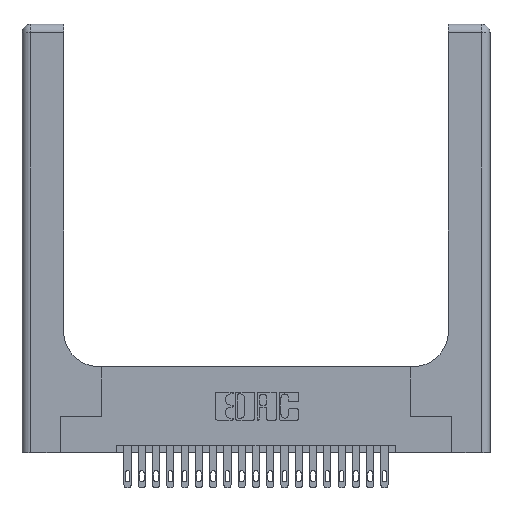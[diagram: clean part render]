
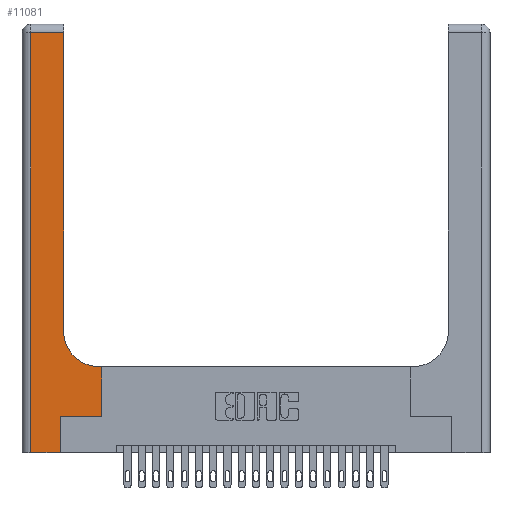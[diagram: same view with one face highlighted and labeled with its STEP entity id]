
A CAD part, top view. The second image highlights one B-rep face of the part: STEP entity #11081.
In plain terms, the highlighted planar face has unit normal (0, 0, 1).
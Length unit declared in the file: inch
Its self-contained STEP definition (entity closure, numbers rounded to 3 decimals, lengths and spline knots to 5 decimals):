
#59 = ORIENTED_EDGE ( 'NONE', *, *, #13412, .T. ) ;
#253 = CARTESIAN_POINT ( 'NONE',  ( 0., 2.94, 0.37 ) ) ;
#1457 = CARTESIAN_POINT ( 'NONE',  ( 0.2915, 2.94, 0.37 ) ) ;
#2071 = CARTESIAN_POINT ( 'NONE',  ( 0.5585, 0.6, 0.37 ) ) ;
#2185 = CARTESIAN_POINT ( 'NONE',  ( 0.5415, 0.6, 0.37 ) ) ;
#2238 = EDGE_CURVE ( 'NONE', #10053, #17259, #12830, .T. ) ;
#3001 = ORIENTED_EDGE ( 'NONE', *, *, #6659, .T. ) ;
#3603 = CARTESIAN_POINT ( 'NONE',  ( 0.269, 0., 0.37 ) ) ;
#3827 = FACE_OUTER_BOUND ( 'NONE', #9935, .T. ) ;
#4841 = VERTEX_POINT ( 'NONE', #17805 ) ;
#5040 = VERTEX_POINT ( 'NONE', #8420 ) ;
#5217 = DIRECTION ( 'NONE',  ( 0., 1., 0. ) ) ;
#5229 = CARTESIAN_POINT ( 'NONE',  ( 0.06, 3., 0.37 ) ) ;
#5377 = CARTESIAN_POINT ( 'NONE',  ( 0.2915, 3., 0.37 ) ) ;
#5409 = CIRCLE ( 'NONE', #11864, 0.25 ) ;
#5424 = LINE ( 'NONE', #3603, #9628 ) ;
#6062 = CARTESIAN_POINT ( 'NONE',  ( 0.2915, 0.6, 0.37 ) ) ;
#6175 = VECTOR ( 'NONE', #8899, 39.37008 ) ;
#6198 = ORIENTED_EDGE ( 'NONE', *, *, #6596, .T. ) ;
#6596 = EDGE_CURVE ( 'NONE', #20016, #17324, #19486, .T. ) ;
#6659 = EDGE_CURVE ( 'NONE', #17259, #13759, #12178, .T. ) ;
#6772 = DIRECTION ( 'NONE',  ( 1., 0., 0. ) ) ;
#7160 = ORIENTED_EDGE ( 'NONE', *, *, #2238, .T. ) ;
#7655 = VECTOR ( 'NONE', #11675, 39.37008 ) ;
#8056 = DIRECTION ( 'NONE',  ( 0., 0., -1. ) ) ;
#8376 = CARTESIAN_POINT ( 'NONE',  ( 0.269, 0.25, 0.37 ) ) ;
#8420 = CARTESIAN_POINT ( 'NONE',  ( 0.2915, 0.85, 0.37 ) ) ;
#8554 = CARTESIAN_POINT ( 'NONE',  ( 0.269, 0.25, 0.37 ) ) ;
#8706 = LINE ( 'NONE', #8554, #6175 ) ;
#8770 = DIRECTION ( 'NONE',  ( 0., 1., 0. ) ) ;
#8836 = CARTESIAN_POINT ( 'NONE',  ( 0.5585, 0.25, 0.37 ) ) ;
#8899 = DIRECTION ( 'NONE',  ( 1., 0., 0. ) ) ;
#9628 = VECTOR ( 'NONE', #17928, 39.37008 ) ;
#9935 = EDGE_LOOP ( 'NONE', ( #18010, #6198, #17158, #59, #19633, #19259, #7160, #3001, #22513 ) ) ;
#10001 = VECTOR ( 'NONE', #16297, 39.37008 ) ;
#10053 = VERTEX_POINT ( 'NONE', #20796 ) ;
#10273 = DIRECTION ( 'NONE',  ( 0., 0., -1. ) ) ;
#10419 = LINE ( 'NONE', #5229, #20478 ) ;
#11081 = ADVANCED_FACE ( 'NONE', ( #3827 ), #20843, .F. ) ;
#11435 = VECTOR ( 'NONE', #5217, 39.37008 ) ;
#11675 = DIRECTION ( 'NONE',  ( 1., 0., 0. ) ) ;
#11835 = VECTOR ( 'NONE', #8770, 39.37008 ) ;
#11864 = AXIS2_PLACEMENT_3D ( 'NONE', #12199, #10273, #6772 ) ;
#12178 = LINE ( 'NONE', #6062, #20592 ) ;
#12199 = CARTESIAN_POINT ( 'NONE',  ( 0.5415, 0.85, 0.37 ) ) ;
#12830 = LINE ( 'NONE', #8836, #11435 ) ;
#13091 = EDGE_CURVE ( 'NONE', #4841, #15959, #5424, .T. ) ;
#13284 = DIRECTION ( 'NONE',  ( -1., 0., 0. ) ) ;
#13308 = CARTESIAN_POINT ( 'NONE',  ( 0., 0., 0.37 ) ) ;
#13412 = EDGE_CURVE ( 'NONE', #21065, #4841, #17661, .T. ) ;
#13606 = DIRECTION ( 'NONE',  ( -1., 0., 0. ) ) ;
#13620 = EDGE_CURVE ( 'NONE', #17324, #21065, #10419, .T. ) ;
#13759 = VERTEX_POINT ( 'NONE', #2185 ) ;
#14146 = EDGE_CURVE ( 'NONE', #13759, #5040, #5409, .T. ) ;
#14644 = CARTESIAN_POINT ( 'NONE',  ( 0.06, 2.94, 0.37 ) ) ;
#15644 = EDGE_CURVE ( 'NONE', #15959, #10053, #8706, .T. ) ;
#15959 = VERTEX_POINT ( 'NONE', #8376 ) ;
#16297 = DIRECTION ( 'NONE',  ( -1., 0., 0. ) ) ;
#17158 = ORIENTED_EDGE ( 'NONE', *, *, #13620, .T. ) ;
#17259 = VERTEX_POINT ( 'NONE', #2071 ) ;
#17324 = VERTEX_POINT ( 'NONE', #14644 ) ;
#17511 = DIRECTION ( 'NONE',  ( 0., -1., 0. ) ) ;
#17661 = LINE ( 'NONE', #13308, #7655 ) ;
#17805 = CARTESIAN_POINT ( 'NONE',  ( 0.269, 0., 0.37 ) ) ;
#17928 = DIRECTION ( 'NONE',  ( 0., 1., 0. ) ) ;
#18010 = ORIENTED_EDGE ( 'NONE', *, *, #18873, .T. ) ;
#18111 = AXIS2_PLACEMENT_3D ( 'NONE', #22402, #8056, #13606 ) ;
#18708 = CARTESIAN_POINT ( 'NONE',  ( 0.06, 0., 0.37 ) ) ;
#18873 = EDGE_CURVE ( 'NONE', #5040, #20016, #21655, .T. ) ;
#19259 = ORIENTED_EDGE ( 'NONE', *, *, #15644, .T. ) ;
#19486 = LINE ( 'NONE', #253, #10001 ) ;
#19633 = ORIENTED_EDGE ( 'NONE', *, *, #13091, .T. ) ;
#20016 = VERTEX_POINT ( 'NONE', #1457 ) ;
#20478 = VECTOR ( 'NONE', #17511, 39.37008 ) ;
#20592 = VECTOR ( 'NONE', #13284, 39.37008 ) ;
#20796 = CARTESIAN_POINT ( 'NONE',  ( 0.5585, 0.25, 0.37 ) ) ;
#20843 = PLANE ( 'NONE',  #18111 ) ;
#21065 = VERTEX_POINT ( 'NONE', #18708 ) ;
#21655 = LINE ( 'NONE', #5377, #11835 ) ;
#22402 = CARTESIAN_POINT ( 'NONE',  ( 0., 3., 0.37 ) ) ;
#22513 = ORIENTED_EDGE ( 'NONE', *, *, #14146, .T. ) ;
